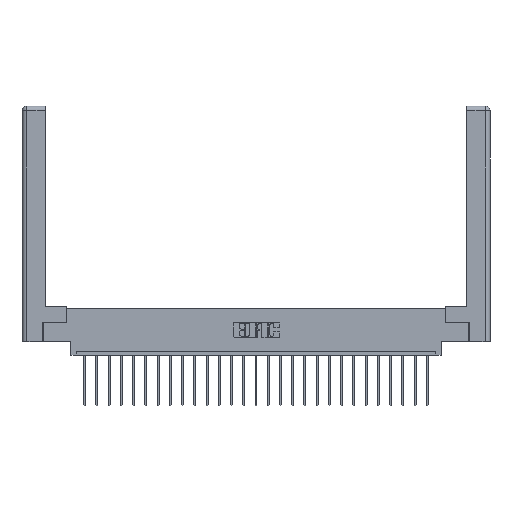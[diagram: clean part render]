
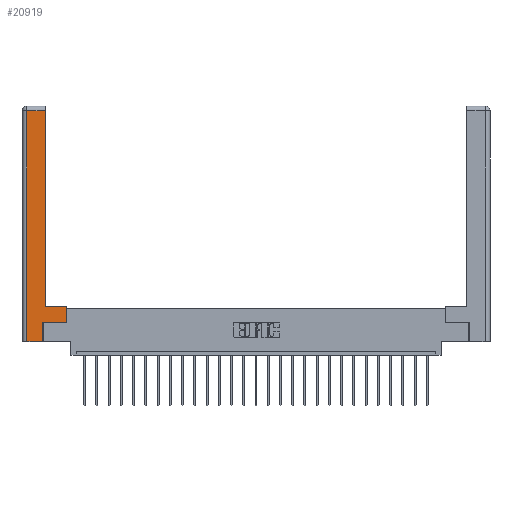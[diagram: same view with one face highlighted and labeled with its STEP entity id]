
A CAD part, top view. The second image highlights one B-rep face of the part: STEP entity #20919.
In plain terms, the highlighted planar face has unit normal (0, 0, 1).
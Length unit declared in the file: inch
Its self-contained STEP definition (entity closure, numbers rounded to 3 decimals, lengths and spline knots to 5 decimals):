
#23 = EDGE_CURVE ( 'NONE', #21346, #24849, #23214, .T. ) ;
#578 = EDGE_CURVE ( 'NONE', #6680, #14234, #4656, .T. ) ;
#851 = ORIENTED_EDGE ( 'NONE', *, *, #907, .T. ) ;
#907 = EDGE_CURVE ( 'NONE', #9209, #25759, #3719, .T. ) ;
#1751 = CARTESIAN_POINT ( 'NONE',  ( 0.0615, 0., 0. ) ) ;
#2327 = LINE ( 'NONE', #13924, #7039 ) ;
#2483 = VECTOR ( 'NONE', #19942, 39.37008 ) ;
#2848 = CARTESIAN_POINT ( 'NONE',  ( 0.295, 0.45, 0. ) ) ;
#2926 = EDGE_CURVE ( 'NONE', #15086, #21346, #2327, .T. ) ;
#3096 = LINE ( 'NONE', #1751, #16304 ) ;
#3132 = CARTESIAN_POINT ( 'NONE',  ( 0.265, 0.245, 0. ) ) ;
#3158 = DIRECTION ( 'NONE',  ( -1., 0., 0. ) ) ;
#3291 = ORIENTED_EDGE ( 'NONE', *, *, #16237, .T. ) ;
#3608 = EDGE_CURVE ( 'NONE', #14234, #17519, #8230, .T. ) ;
#3719 = LINE ( 'NONE', #21419, #6847 ) ;
#4656 = LINE ( 'NONE', #22174, #9703 ) ;
#4823 = ORIENTED_EDGE ( 'NONE', *, *, #578, .T. ) ;
#6680 = VERTEX_POINT ( 'NONE', #2848 ) ;
#6847 = VECTOR ( 'NONE', #23260, 39.37008 ) ;
#7039 = VECTOR ( 'NONE', #26016, 39.37008 ) ;
#7269 = EDGE_CURVE ( 'NONE', #25759, #15086, #11142, .T. ) ;
#7796 = DIRECTION ( 'NONE',  ( 0., 1., 0. ) ) ;
#7887 = CARTESIAN_POINT ( 'NONE',  ( 0.265, 0.245, 0. ) ) ;
#8230 = LINE ( 'NONE', #16768, #23636 ) ;
#8338 = AXIS2_PLACEMENT_3D ( 'NONE', #15187, #15089, #3158 ) ;
#8679 = CARTESIAN_POINT ( 'NONE',  ( 0.0615, 0., 0. ) ) ;
#9209 = VERTEX_POINT ( 'NONE', #8679 ) ;
#9703 = VECTOR ( 'NONE', #14010, 39.37008 ) ;
#9864 = ORIENTED_EDGE ( 'NONE', *, *, #23, .T. ) ;
#10692 = ORIENTED_EDGE ( 'NONE', *, *, #3608, .T. ) ;
#10833 = VECTOR ( 'NONE', #7796, 39.37008 ) ;
#11063 = PLANE ( 'NONE',  #8338 ) ;
#11142 = LINE ( 'NONE', #7887, #10833 ) ;
#13120 = CARTESIAN_POINT ( 'NONE',  ( 0.565, 0.245, 0. ) ) ;
#13924 = CARTESIAN_POINT ( 'NONE',  ( 0.565, 0.245, 0. ) ) ;
#14010 = DIRECTION ( 'NONE',  ( 0., 1., 0. ) ) ;
#14234 = VERTEX_POINT ( 'NONE', #20547 ) ;
#14823 = ORIENTED_EDGE ( 'NONE', *, *, #7269, .T. ) ;
#15086 = VERTEX_POINT ( 'NONE', #3132 ) ;
#15089 = DIRECTION ( 'NONE',  ( 0., 0., -1. ) ) ;
#15187 = CARTESIAN_POINT ( 'NONE',  ( 0., 0., 0. ) ) ;
#15438 = ORIENTED_EDGE ( 'NONE', *, *, #2926, .T. ) ;
#15798 = ORIENTED_EDGE ( 'NONE', *, *, #22637, .T. ) ;
#16237 = EDGE_CURVE ( 'NONE', #24849, #6680, #24781, .T. ) ;
#16304 = VECTOR ( 'NONE', #19606, 39.37008 ) ;
#16768 = CARTESIAN_POINT ( 'NONE',  ( 0.0615, 2.94, 0. ) ) ;
#17519 = VERTEX_POINT ( 'NONE', #21589 ) ;
#18682 = CARTESIAN_POINT ( 'NONE',  ( 0.295, 0.45, 0. ) ) ;
#18830 = VECTOR ( 'NONE', #24705, 39.37008 ) ;
#18931 = FACE_OUTER_BOUND ( 'NONE', #22739, .T. ) ;
#19606 = DIRECTION ( 'NONE',  ( 0., -1., 0. ) ) ;
#19942 = DIRECTION ( 'NONE',  ( 0., 1., 0. ) ) ;
#20186 = CARTESIAN_POINT ( 'NONE',  ( 0.565, 0.45, 0. ) ) ;
#20547 = CARTESIAN_POINT ( 'NONE',  ( 0.295, 2.94, 0. ) ) ;
#20919 = ADVANCED_FACE ( 'NONE', ( #18931 ), #11063, .F. ) ;
#21346 = VERTEX_POINT ( 'NONE', #13120 ) ;
#21419 = CARTESIAN_POINT ( 'NONE',  ( 0.265, 0., 0. ) ) ;
#21589 = CARTESIAN_POINT ( 'NONE',  ( 0.0615, 2.94, 0. ) ) ;
#22174 = CARTESIAN_POINT ( 'NONE',  ( 0.295, 3., 0. ) ) ;
#22637 = EDGE_CURVE ( 'NONE', #17519, #9209, #3096, .T. ) ;
#22739 = EDGE_LOOP ( 'NONE', ( #4823, #10692, #15798, #851, #14823, #15438, #9864, #3291 ) ) ;
#23214 = LINE ( 'NONE', #20186, #2483 ) ;
#23260 = DIRECTION ( 'NONE',  ( 1., 0., 0. ) ) ;
#23636 = VECTOR ( 'NONE', #24903, 39.37008 ) ;
#24705 = DIRECTION ( 'NONE',  ( -1., 0., 0. ) ) ;
#24781 = LINE ( 'NONE', #18682, #18830 ) ;
#24849 = VERTEX_POINT ( 'NONE', #25559 ) ;
#24903 = DIRECTION ( 'NONE',  ( -1., 0., 0. ) ) ;
#24938 = CARTESIAN_POINT ( 'NONE',  ( 0.265, 0., 0. ) ) ;
#25559 = CARTESIAN_POINT ( 'NONE',  ( 0.565, 0.45, 0. ) ) ;
#25759 = VERTEX_POINT ( 'NONE', #24938 ) ;
#26016 = DIRECTION ( 'NONE',  ( 1., 0., 0. ) ) ;
